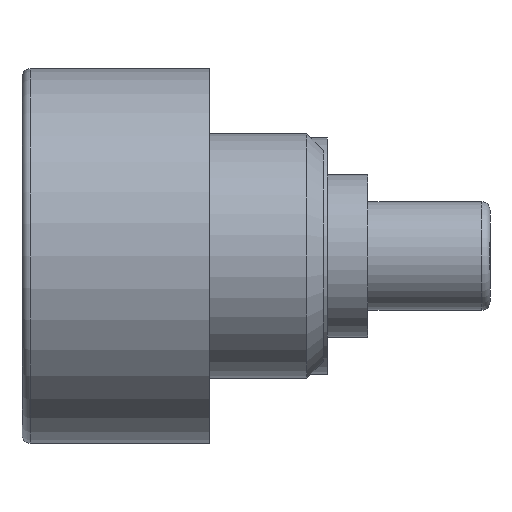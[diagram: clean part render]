
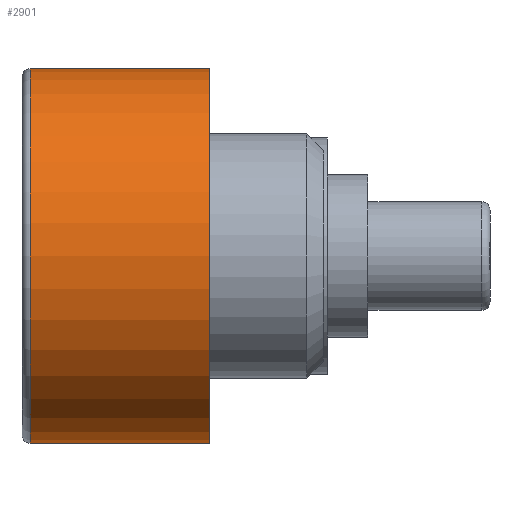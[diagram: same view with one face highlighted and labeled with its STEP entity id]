
A CAD part, left-side view. The second image highlights one B-rep face of the part: STEP entity #2901.
In plain terms, the highlighted cylindrical face has radius 2.3 mm (diameter 4.6 mm), a partial arc.
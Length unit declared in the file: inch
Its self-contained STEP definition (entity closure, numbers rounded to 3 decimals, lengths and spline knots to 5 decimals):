
#132 = DIRECTION ( 'NONE',  ( 0., 1., 0. ) ) ;
#161 = DIRECTION ( 'NONE',  ( 0., 0., 1. ) ) ;
#164 = AXIS2_PLACEMENT_3D ( 'NONE', #4361, #132, #2299 ) ;
#197 = FACE_OUTER_BOUND ( 'NONE', #1372, .T. ) ;
#262 = EDGE_CURVE ( 'NONE', #2476, #5092, #529, .T. ) ;
#333 = CARTESIAN_POINT ( 'NONE',  ( -0.2878, 0.04134, -0.09055 ) ) ;
#529 = LINE ( 'NONE', #6416, #5877 ) ;
#752 = DIRECTION ( 'NONE',  ( 0., -1., 0. ) ) ;
#820 = DIRECTION ( 'NONE',  ( 0., 0., 1. ) ) ;
#993 = ORIENTED_EDGE ( 'NONE', *, *, #3379, .T. ) ;
#1140 = CARTESIAN_POINT ( 'NONE',  ( -0.2878, -0.04528, 0.09055 ) ) ;
#1216 = CARTESIAN_POINT ( 'NONE',  ( -0.2878, 0.04134, 0.09055 ) ) ;
#1263 = ORIENTED_EDGE ( 'NONE', *, *, #1771, .T. ) ;
#1367 = VERTEX_POINT ( 'NONE', #1140 ) ;
#1372 = EDGE_LOOP ( 'NONE', ( #1263, #993, #5870, #2517 ) ) ;
#1385 = DIRECTION ( 'NONE',  ( 0., 1., 0. ) ) ;
#1771 = EDGE_CURVE ( 'NONE', #1367, #4103, #4551, .T. ) ;
#1945 = AXIS2_PLACEMENT_3D ( 'NONE', #5483, #6542, #161 ) ;
#2172 = CARTESIAN_POINT ( 'NONE',  ( -0.2878, -0.04528, -0.09055 ) ) ;
#2299 = DIRECTION ( 'NONE',  ( 0., 0., 1. ) ) ;
#2476 = VERTEX_POINT ( 'NONE', #2172 ) ;
#2517 = ORIENTED_EDGE ( 'NONE', *, *, #2920, .T. ) ;
#2901 = ADVANCED_FACE ( 'NONE', ( #197 ), #5964, .T. ) ;
#2920 = EDGE_CURVE ( 'NONE', #2476, #1367, #3182, .T. ) ;
#3182 = CIRCLE ( 'NONE', #164, 0.09055 ) ;
#3313 = CIRCLE ( 'NONE', #6560, 0.09055 ) ;
#3358 = VECTOR ( 'NONE', #1385, 39.37008 ) ;
#3379 = EDGE_CURVE ( 'NONE', #4103, #5092, #3313, .T. ) ;
#4070 = CARTESIAN_POINT ( 'NONE',  ( -0.2878, -0.04528, 0.09055 ) ) ;
#4103 = VERTEX_POINT ( 'NONE', #1216 ) ;
#4361 = CARTESIAN_POINT ( 'NONE',  ( -0.2878, -0.04528, 0. ) ) ;
#4551 = LINE ( 'NONE', #4070, #3358 ) ;
#4848 = DIRECTION ( 'NONE',  ( 0., 1., 0. ) ) ;
#5092 = VERTEX_POINT ( 'NONE', #333 ) ;
#5483 = CARTESIAN_POINT ( 'NONE',  ( -0.2878, -0.04528, 0. ) ) ;
#5571 = CARTESIAN_POINT ( 'NONE',  ( -0.2878, 0.04134, 0. ) ) ;
#5870 = ORIENTED_EDGE ( 'NONE', *, *, #262, .F. ) ;
#5877 = VECTOR ( 'NONE', #4848, 39.37008 ) ;
#5964 = CYLINDRICAL_SURFACE ( 'NONE', #1945, 0.09055 ) ;
#6416 = CARTESIAN_POINT ( 'NONE',  ( -0.2878, -0.04528, -0.09055 ) ) ;
#6542 = DIRECTION ( 'NONE',  ( 0., 1., 0. ) ) ;
#6560 = AXIS2_PLACEMENT_3D ( 'NONE', #5571, #752, #820 ) ;
